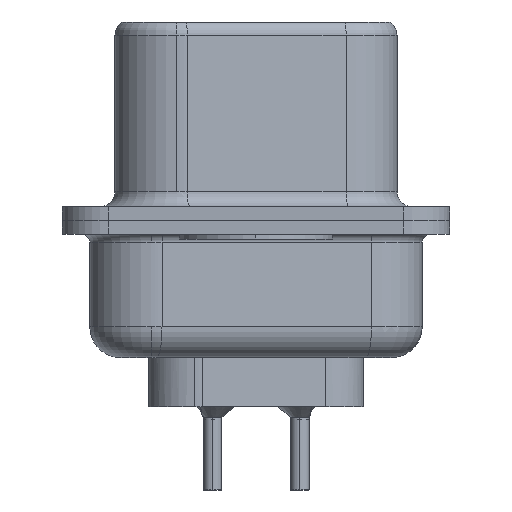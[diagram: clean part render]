
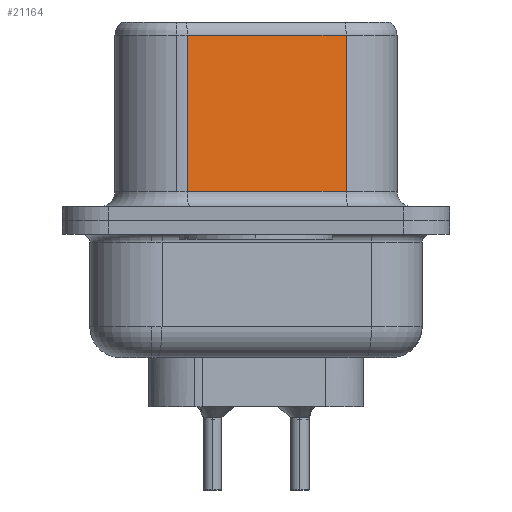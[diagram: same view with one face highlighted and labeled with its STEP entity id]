
A CAD part, left-side view. The second image highlights one B-rep face of the part: STEP entity #21164.
In plain terms, the highlighted planar face has unit normal (-0.985, -0.174, 0).
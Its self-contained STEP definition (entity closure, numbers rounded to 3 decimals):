
#1567 = EDGE_CURVE ( 'NONE', #16818, #20859, #12802, .T. ) ;
#1856 = VECTOR ( 'NONE', #3714, 1000. ) ;
#3206 = FACE_OUTER_BOUND ( 'NONE', #10186, .T. ) ;
#3714 = DIRECTION ( 'NONE',  ( -0.174, 0.985, 0. ) ) ;
#3771 = DIRECTION ( 'NONE',  ( 0.174, -0.985, 0. ) ) ;
#3896 = CARTESIAN_POINT ( 'NONE',  ( 3.67, 2.233, 0.95 ) ) ;
#4118 = EDGE_CURVE ( 'NONE', #7885, #16818, #16376, .T. ) ;
#4206 = ORIENTED_EDGE ( 'NONE', *, *, #8337, .F. ) ;
#5084 = CARTESIAN_POINT ( 'NONE',  ( 4.58, -2.927, 6.52 ) ) ;
#5821 = CARTESIAN_POINT ( 'NONE',  ( 4.58, -2.927, 0.95 ) ) ;
#6754 = DIRECTION ( 'NONE',  ( 0.985, 0.174, 0. ) ) ;
#7305 = CARTESIAN_POINT ( 'NONE',  ( 3.67, 2.233, 6.02 ) ) ;
#7560 = AXIS2_PLACEMENT_3D ( 'NONE', #11926, #6754, #19324 ) ;
#7885 = VERTEX_POINT ( 'NONE', #7305 ) ;
#8337 = EDGE_CURVE ( 'NONE', #21451, #20859, #20739, .T. ) ;
#8740 = ORIENTED_EDGE ( 'NONE', *, *, #1567, .T. ) ;
#9537 = EDGE_CURVE ( 'NONE', #21451, #7885, #17308, .T. ) ;
#10186 = EDGE_LOOP ( 'NONE', ( #4206, #12260, #15794, #8740 ) ) ;
#11046 = CARTESIAN_POINT ( 'NONE',  ( 4.58, -2.927, 6.02 ) ) ;
#11522 = VECTOR ( 'NONE', #17861, 1000. ) ;
#11926 = CARTESIAN_POINT ( 'NONE',  ( 4.58, -2.927, 6.52 ) ) ;
#12149 = CARTESIAN_POINT ( 'NONE',  ( 4.58, -2.927, 0.95 ) ) ;
#12260 = ORIENTED_EDGE ( 'NONE', *, *, #9537, .T. ) ;
#12802 = LINE ( 'NONE', #12149, #21319 ) ;
#13986 = DIRECTION ( 'NONE',  ( 0., 0., -1. ) ) ;
#15794 = ORIENTED_EDGE ( 'NONE', *, *, #4118, .T. ) ;
#16376 = LINE ( 'NONE', #23206, #11522 ) ;
#16818 = VERTEX_POINT ( 'NONE', #3896 ) ;
#17308 = LINE ( 'NONE', #21627, #1856 ) ;
#17485 = PLANE ( 'NONE',  #7560 ) ;
#17861 = DIRECTION ( 'NONE',  ( 0., 0., -1. ) ) ;
#19324 = DIRECTION ( 'NONE',  ( -0.174, 0.985, 0. ) ) ;
#20179 = VECTOR ( 'NONE', #13986, 1000. ) ;
#20739 = LINE ( 'NONE', #5084, #20179 ) ;
#20859 = VERTEX_POINT ( 'NONE', #5821 ) ;
#21164 = ADVANCED_FACE ( 'NONE', ( #3206 ), #17485, .F. ) ;
#21319 = VECTOR ( 'NONE', #3771, 1000. ) ;
#21451 = VERTEX_POINT ( 'NONE', #11046 ) ;
#21627 = CARTESIAN_POINT ( 'NONE',  ( 4.58, -2.927, 6.02 ) ) ;
#23206 = CARTESIAN_POINT ( 'NONE',  ( 3.67, 2.233, 6.52 ) ) ;
